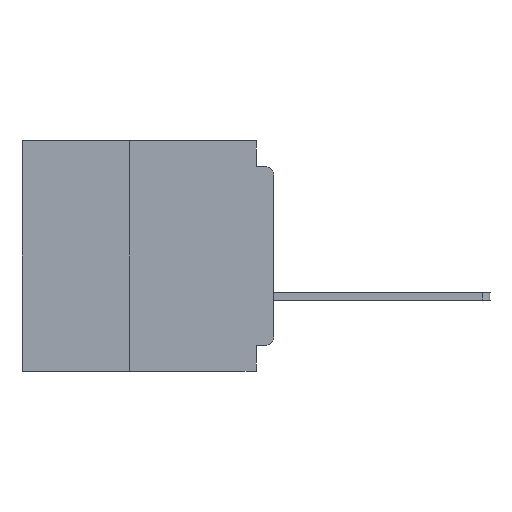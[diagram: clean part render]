
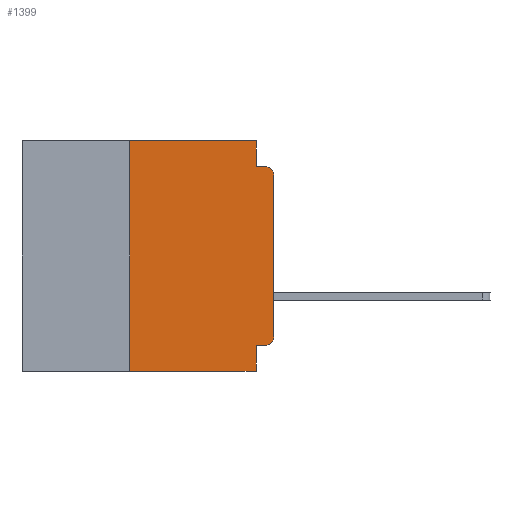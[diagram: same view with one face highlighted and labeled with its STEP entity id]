
A CAD part, left-side view. The second image highlights one B-rep face of the part: STEP entity #1399.
In plain terms, the highlighted planar face has unit normal (-1, 0, 0).
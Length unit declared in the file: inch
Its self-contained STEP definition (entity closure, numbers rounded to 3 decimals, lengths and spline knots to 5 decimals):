
#129 = LINE ( 'NONE', #36087, #53258 ) ;
#1399 = ADVANCED_FACE ( 'NONE', ( #26952 ), #59773, .F. ) ;
#1547 = ORIENTED_EDGE ( 'NONE', *, *, #25965, .F. ) ;
#1857 = DIRECTION ( 'NONE',  ( -1., 0., 0. ) ) ;
#2045 = DIRECTION ( 'NONE',  ( -1., 0., 0. ) ) ;
#2971 = LINE ( 'NONE', #34960, #15097 ) ;
#3136 = CARTESIAN_POINT ( 'NONE',  ( 0., 0.25, -0.4 ) ) ;
#5262 = DIRECTION ( 'NONE',  ( 0., -1., 0. ) ) ;
#6239 = VECTOR ( 'NONE', #44259, 39.37008 ) ;
#7112 = CARTESIAN_POINT ( 'NONE',  ( 0., 0.015, -0.355 ) ) ;
#7544 = EDGE_CURVE ( 'NONE', #51551, #25920, #13311, .T. ) ;
#9067 = CARTESIAN_POINT ( 'NONE',  ( 0., 0.25, -0.4 ) ) ;
#9551 = DIRECTION ( 'NONE',  ( 0., -1., 0. ) ) ;
#9942 = LINE ( 'NONE', #13280, #46093 ) ;
#10053 = CARTESIAN_POINT ( 'NONE',  ( 0., 0.031, -0.355 ) ) ;
#11594 = CARTESIAN_POINT ( 'NONE',  ( 0., 0., -0.355 ) ) ;
#12269 = EDGE_LOOP ( 'NONE', ( #56443, #30073, #62111, #20180, #57290, #29734, #40656, #1547, #38028, #31369 ) ) ;
#12683 = EDGE_CURVE ( 'NONE', #43379, #66250, #2971, .T. ) ;
#13280 = CARTESIAN_POINT ( 'NONE',  ( 0., 0.031, -0.4 ) ) ;
#13311 = LINE ( 'NONE', #43139, #54257 ) ;
#13823 = CARTESIAN_POINT ( 'NONE',  ( 0., 0.031, -0.045 ) ) ;
#15097 = VECTOR ( 'NONE', #9551, 39.37008 ) ;
#16170 = LINE ( 'NONE', #54121, #53847 ) ;
#20180 = ORIENTED_EDGE ( 'NONE', *, *, #35348, .F. ) ;
#21138 = VECTOR ( 'NONE', #47493, 39.37008 ) ;
#21517 = CARTESIAN_POINT ( 'NONE',  ( 0., 0.031, 0. ) ) ;
#25920 = VERTEX_POINT ( 'NONE', #33515 ) ;
#25965 = EDGE_CURVE ( 'NONE', #50413, #55670, #9942, .T. ) ;
#26018 = DIRECTION ( 'NONE',  ( 0., 0., -1. ) ) ;
#26952 = FACE_OUTER_BOUND ( 'NONE', #12269, .T. ) ;
#27010 = EDGE_CURVE ( 'NONE', #57257, #50413, #34707, .T. ) ;
#29734 = ORIENTED_EDGE ( 'NONE', *, *, #55927, .F. ) ;
#30073 = ORIENTED_EDGE ( 'NONE', *, *, #57880, .T. ) ;
#31369 = ORIENTED_EDGE ( 'NONE', *, *, #53217, .T. ) ;
#32733 = CARTESIAN_POINT ( 'NONE',  ( 0., 0.015, -0.34 ) ) ;
#32915 = CARTESIAN_POINT ( 'NONE',  ( 0., 0.015, -0.06 ) ) ;
#33515 = CARTESIAN_POINT ( 'NONE',  ( 0., 0.015, -0.045 ) ) ;
#34707 = LINE ( 'NONE', #11594, #21138 ) ;
#34960 = CARTESIAN_POINT ( 'NONE',  ( 0., 0.437, 0. ) ) ;
#35199 = LINE ( 'NONE', #3136, #6239 ) ;
#35348 = EDGE_CURVE ( 'NONE', #66250, #51551, #42376, .T. ) ;
#36087 = CARTESIAN_POINT ( 'NONE',  ( 0., 0.437, -0.4 ) ) ;
#36192 = CARTESIAN_POINT ( 'NONE',  ( 0., 0.25, 0. ) ) ;
#36456 = AXIS2_PLACEMENT_3D ( 'NONE', #60478, #57859, #57335 ) ;
#37872 = DIRECTION ( 'NONE',  ( 0., 0., -1. ) ) ;
#38028 = ORIENTED_EDGE ( 'NONE', *, *, #27010, .F. ) ;
#38047 = DIRECTION ( 'NONE',  ( 0., 0., -1. ) ) ;
#38443 = CIRCLE ( 'NONE', #41492, 0.015 ) ;
#40656 = ORIENTED_EDGE ( 'NONE', *, *, #40940, .T. ) ;
#40751 = VECTOR ( 'NONE', #26018, 39.37008 ) ;
#40940 = EDGE_CURVE ( 'NONE', #47398, #55670, #129, .T. ) ;
#41492 = AXIS2_PLACEMENT_3D ( 'NONE', #32733, #1857, #37872 ) ;
#42316 = CARTESIAN_POINT ( 'NONE',  ( 0., 0., -0.06 ) ) ;
#42376 = LINE ( 'NONE', #56635, #40751 ) ;
#43139 = CARTESIAN_POINT ( 'NONE',  ( 0., 0., -0.045 ) ) ;
#43379 = VERTEX_POINT ( 'NONE', #36192 ) ;
#44259 = DIRECTION ( 'NONE',  ( 0., 0., 1. ) ) ;
#46093 = VECTOR ( 'NONE', #54337, 39.37008 ) ;
#47398 = VERTEX_POINT ( 'NONE', #9067 ) ;
#47493 = DIRECTION ( 'NONE',  ( 0., 1., 0. ) ) ;
#48276 = DIRECTION ( 'NONE',  ( 0., -1., 0. ) ) ;
#48537 = VERTEX_POINT ( 'NONE', #50240 ) ;
#48961 = DIRECTION ( 'NONE',  ( 0., 0., 1. ) ) ;
#49342 = CIRCLE ( 'NONE', #51646, 0.015 ) ;
#50240 = CARTESIAN_POINT ( 'NONE',  ( 0., 0., -0.34 ) ) ;
#50413 = VERTEX_POINT ( 'NONE', #10053 ) ;
#51551 = VERTEX_POINT ( 'NONE', #13823 ) ;
#51646 = AXIS2_PLACEMENT_3D ( 'NONE', #32915, #2045, #38047 ) ;
#51899 = VERTEX_POINT ( 'NONE', #42316 ) ;
#53217 = EDGE_CURVE ( 'NONE', #57257, #48537, #38443, .T. ) ;
#53258 = VECTOR ( 'NONE', #5262, 39.37008 ) ;
#53847 = VECTOR ( 'NONE', #48961, 39.37008 ) ;
#54121 = CARTESIAN_POINT ( 'NONE',  ( 0., 0., 0. ) ) ;
#54257 = VECTOR ( 'NONE', #48276, 39.37008 ) ;
#54337 = DIRECTION ( 'NONE',  ( 0., 0., -1. ) ) ;
#55670 = VERTEX_POINT ( 'NONE', #57714 ) ;
#55927 = EDGE_CURVE ( 'NONE', #47398, #43379, #35199, .T. ) ;
#56443 = ORIENTED_EDGE ( 'NONE', *, *, #62120, .T. ) ;
#56635 = CARTESIAN_POINT ( 'NONE',  ( 0., 0.031, 0. ) ) ;
#57257 = VERTEX_POINT ( 'NONE', #7112 ) ;
#57290 = ORIENTED_EDGE ( 'NONE', *, *, #12683, .F. ) ;
#57335 = DIRECTION ( 'NONE',  ( 0., 0., -1. ) ) ;
#57714 = CARTESIAN_POINT ( 'NONE',  ( 0., 0.031, -0.4 ) ) ;
#57859 = DIRECTION ( 'NONE',  ( 1., 0., 0. ) ) ;
#57880 = EDGE_CURVE ( 'NONE', #51899, #25920, #49342, .T. ) ;
#59773 = PLANE ( 'NONE',  #36456 ) ;
#60478 = CARTESIAN_POINT ( 'NONE',  ( 0., 0.437, 0. ) ) ;
#62111 = ORIENTED_EDGE ( 'NONE', *, *, #7544, .F. ) ;
#62120 = EDGE_CURVE ( 'NONE', #48537, #51899, #16170, .T. ) ;
#66250 = VERTEX_POINT ( 'NONE', #21517 ) ;
